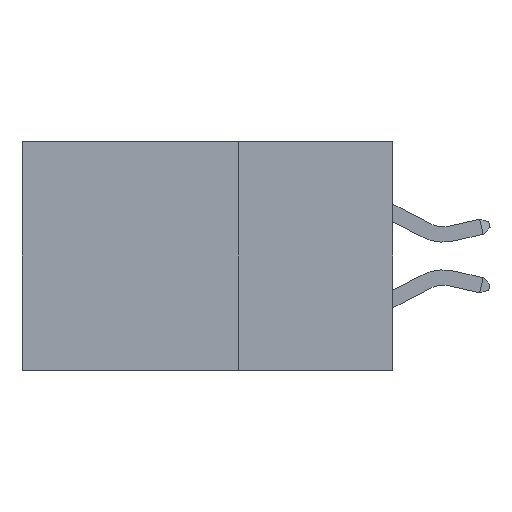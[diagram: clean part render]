
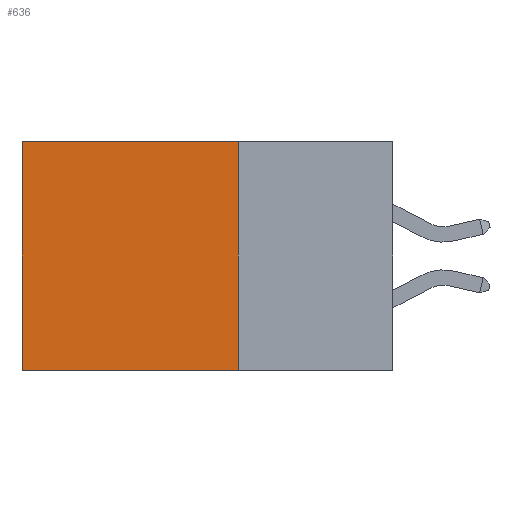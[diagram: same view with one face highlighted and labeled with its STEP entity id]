
A CAD part, left-side view. The second image highlights one B-rep face of the part: STEP entity #636.
In plain terms, the highlighted planar face has unit normal (-1, 0, 0).
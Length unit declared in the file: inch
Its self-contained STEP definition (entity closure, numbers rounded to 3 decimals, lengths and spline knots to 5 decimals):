
#501 = CARTESIAN_POINT ( 'NONE',  ( 0.2875, 0.6, 0. ) ) ;
#609 = CARTESIAN_POINT ( 'NONE',  ( 0.2875, 0.6, 0. ) ) ;
#636 = ADVANCED_FACE ( 'NONE', ( #5221 ), #843, .F. ) ;
#706 = DIRECTION ( 'NONE',  ( 0., 0., -1. ) ) ;
#843 = PLANE ( 'NONE',  #14957 ) ;
#1197 = VECTOR ( 'NONE', #13734, 39.37008 ) ;
#1615 = CARTESIAN_POINT ( 'NONE',  ( 0.2875, 0.25, -0.37 ) ) ;
#1671 = LINE ( 'NONE', #10559, #8054 ) ;
#2392 = EDGE_CURVE ( 'NONE', #3312, #2809, #1671, .T. ) ;
#2809 = VERTEX_POINT ( 'NONE', #6826 ) ;
#3312 = VERTEX_POINT ( 'NONE', #13650 ) ;
#4276 = LINE ( 'NONE', #15095, #10774 ) ;
#4781 = EDGE_CURVE ( 'NONE', #13909, #7949, #5308, .T. ) ;
#5221 = FACE_OUTER_BOUND ( 'NONE', #15411, .T. ) ;
#5308 = LINE ( 'NONE', #609, #8188 ) ;
#5463 = EDGE_CURVE ( 'NONE', #2809, #7949, #7987, .T. ) ;
#6180 = ORIENTED_EDGE ( 'NONE', *, *, #2392, .F. ) ;
#6709 = DIRECTION ( 'NONE',  ( 1., 0., 0. ) ) ;
#6826 = CARTESIAN_POINT ( 'NONE',  ( 0.2875, 0.25, -0.37 ) ) ;
#6841 = DIRECTION ( 'NONE',  ( 0., 0., -1. ) ) ;
#7602 = ORIENTED_EDGE ( 'NONE', *, *, #5463, .F. ) ;
#7949 = VERTEX_POINT ( 'NONE', #15276 ) ;
#7987 = LINE ( 'NONE', #1615, #1197 ) ;
#8054 = VECTOR ( 'NONE', #13810, 39.37008 ) ;
#8188 = VECTOR ( 'NONE', #706, 39.37008 ) ;
#9015 = CARTESIAN_POINT ( 'NONE',  ( 0.2875, 0.25, 0. ) ) ;
#9874 = EDGE_CURVE ( 'NONE', #3312, #13909, #4276, .T. ) ;
#10063 = ORIENTED_EDGE ( 'NONE', *, *, #4781, .T. ) ;
#10559 = CARTESIAN_POINT ( 'NONE',  ( 0.2875, 0.25, 0. ) ) ;
#10688 = DIRECTION ( 'NONE',  ( 0., 1., 0. ) ) ;
#10774 = VECTOR ( 'NONE', #10688, 39.37008 ) ;
#13650 = CARTESIAN_POINT ( 'NONE',  ( 0.2875, 0.25, 0. ) ) ;
#13734 = DIRECTION ( 'NONE',  ( 0., 1., 0. ) ) ;
#13804 = ORIENTED_EDGE ( 'NONE', *, *, #9874, .T. ) ;
#13810 = DIRECTION ( 'NONE',  ( 0., 0., -1. ) ) ;
#13909 = VERTEX_POINT ( 'NONE', #501 ) ;
#14957 = AXIS2_PLACEMENT_3D ( 'NONE', #9015, #6709, #6841 ) ;
#15095 = CARTESIAN_POINT ( 'NONE',  ( 0.2875, 0.25, 0. ) ) ;
#15276 = CARTESIAN_POINT ( 'NONE',  ( 0.2875, 0.6, -0.37 ) ) ;
#15411 = EDGE_LOOP ( 'NONE', ( #10063, #7602, #6180, #13804 ) ) ;
